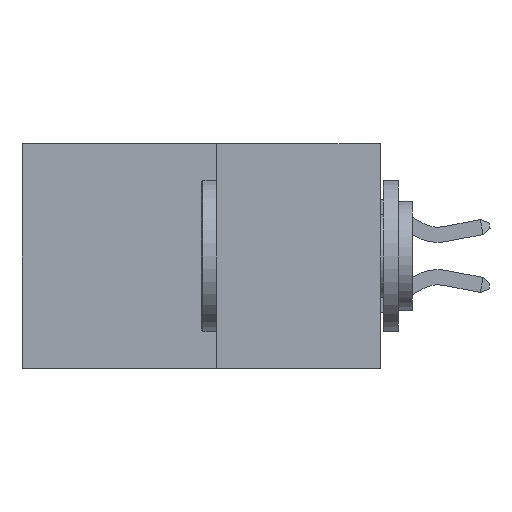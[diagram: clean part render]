
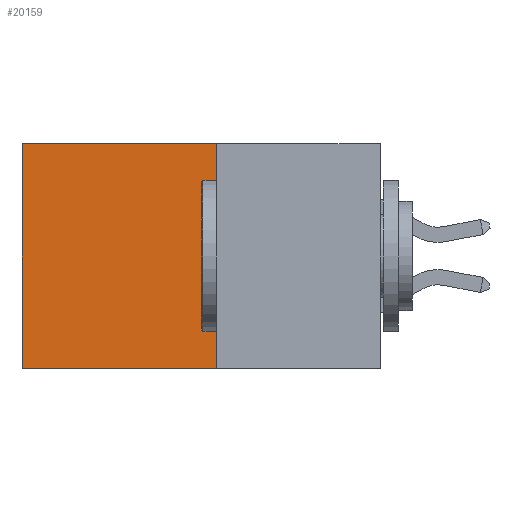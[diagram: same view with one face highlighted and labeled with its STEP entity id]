
A CAD part, left-side view. The second image highlights one B-rep face of the part: STEP entity #20159.
In plain terms, the highlighted planar face has unit normal (-1, 0, 0).
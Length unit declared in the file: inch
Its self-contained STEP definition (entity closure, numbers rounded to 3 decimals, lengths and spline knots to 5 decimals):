
#411 = PLANE ( 'NONE',  #21110 ) ;
#1099 = CARTESIAN_POINT ( 'NONE',  ( 0.277, 0.59, -0.37 ) ) ;
#1449 = VECTOR ( 'NONE', #30279, 39.37008 ) ;
#1548 = CARTESIAN_POINT ( 'NONE',  ( 0.277, 0.59, -0.37 ) ) ;
#2189 = EDGE_CURVE ( 'NONE', #27564, #2459, #20703, .T. ) ;
#2390 = ORIENTED_EDGE ( 'NONE', *, *, #3646, .T. ) ;
#2459 = VERTEX_POINT ( 'NONE', #1548 ) ;
#2547 = CARTESIAN_POINT ( 'NONE',  ( 0.277, 0.27, -0.37 ) ) ;
#2843 = DIRECTION ( 'NONE',  ( 0., 0., -1. ) ) ;
#2891 = CARTESIAN_POINT ( 'NONE',  ( 0.277, 0.27, -0.37 ) ) ;
#3646 = EDGE_CURVE ( 'NONE', #4003, #2459, #30110, .T. ) ;
#4003 = VERTEX_POINT ( 'NONE', #21789 ) ;
#4768 = VECTOR ( 'NONE', #30532, 39.37008 ) ;
#4848 = CARTESIAN_POINT ( 'NONE',  ( 0.277, 0.27, 0. ) ) ;
#5208 = DIRECTION ( 'NONE',  ( 0., 0., -1. ) ) ;
#5594 = LINE ( 'NONE', #2891, #18428 ) ;
#11924 = VERTEX_POINT ( 'NONE', #4848 ) ;
#14678 = CARTESIAN_POINT ( 'NONE',  ( 0.277, 0.27, -0.37 ) ) ;
#15454 = ORIENTED_EDGE ( 'NONE', *, *, #29299, .F. ) ;
#17018 = EDGE_CURVE ( 'NONE', #11924, #4003, #29597, .T. ) ;
#17114 = VECTOR ( 'NONE', #19012, 39.37008 ) ;
#17318 = DIRECTION ( 'NONE',  ( 1., 0., 0. ) ) ;
#17489 = EDGE_LOOP ( 'NONE', ( #2390, #19160, #15454, #22779 ) ) ;
#18428 = VECTOR ( 'NONE', #5208, 39.37008 ) ;
#19012 = DIRECTION ( 'NONE',  ( 0., 1., 0. ) ) ;
#19160 = ORIENTED_EDGE ( 'NONE', *, *, #2189, .F. ) ;
#19595 = CARTESIAN_POINT ( 'NONE',  ( 0.277, 0.27, -0.37 ) ) ;
#20159 = ADVANCED_FACE ( 'NONE', ( #26461 ), #411, .F. ) ;
#20703 = LINE ( 'NONE', #2547, #1449 ) ;
#21110 = AXIS2_PLACEMENT_3D ( 'NONE', #19595, #17318, #2843 ) ;
#21401 = CARTESIAN_POINT ( 'NONE',  ( 0.277, 0.27, 0. ) ) ;
#21789 = CARTESIAN_POINT ( 'NONE',  ( 0.277, 0.59, 0. ) ) ;
#22779 = ORIENTED_EDGE ( 'NONE', *, *, #17018, .T. ) ;
#26461 = FACE_OUTER_BOUND ( 'NONE', #17489, .T. ) ;
#27564 = VERTEX_POINT ( 'NONE', #14678 ) ;
#29299 = EDGE_CURVE ( 'NONE', #11924, #27564, #5594, .T. ) ;
#29597 = LINE ( 'NONE', #21401, #17114 ) ;
#30110 = LINE ( 'NONE', #1099, #4768 ) ;
#30279 = DIRECTION ( 'NONE',  ( 0., 1., 0. ) ) ;
#30532 = DIRECTION ( 'NONE',  ( 0., 0., -1. ) ) ;
